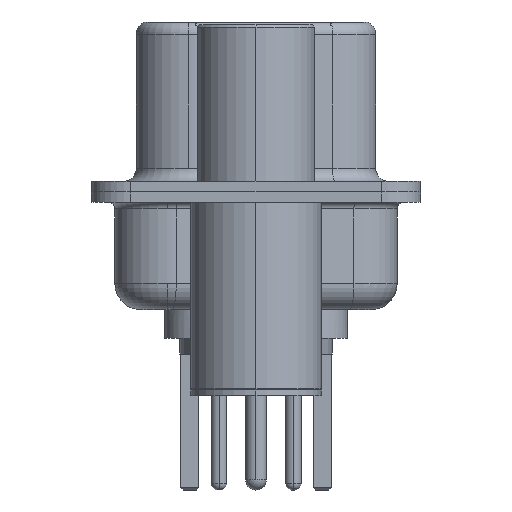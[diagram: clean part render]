
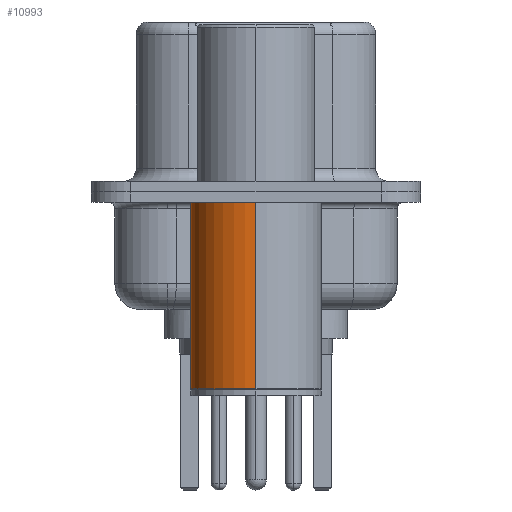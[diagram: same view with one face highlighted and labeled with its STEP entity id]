
A CAD part, left-side view. The second image highlights one B-rep face of the part: STEP entity #10993.
In plain terms, the highlighted cylindrical face has radius 2.5 mm (diameter 5 mm), a partial arc.
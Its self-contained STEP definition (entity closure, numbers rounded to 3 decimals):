
#66 = CARTESIAN_POINT ( 'NONE',  ( 0., 0., -7.525 ) ) ;
#542 = VECTOR ( 'NONE', #2726, 1000. ) ;
#605 = DIRECTION ( 'NONE',  ( 0., 0., 1. ) ) ;
#1313 = EDGE_CURVE ( 'NONE', #32355, #5717, #28626, .T. ) ;
#2302 = DIRECTION ( 'NONE',  ( 0., 0., 1. ) ) ;
#2422 = VERTEX_POINT ( 'NONE', #10895 ) ;
#2499 = ORIENTED_EDGE ( 'NONE', *, *, #11077, .F. ) ;
#2726 = DIRECTION ( 'NONE',  ( 0., 0., 1. ) ) ;
#2835 = CARTESIAN_POINT ( 'NONE',  ( 2.5, 0., -0.4 ) ) ;
#5717 = VERTEX_POINT ( 'NONE', #25246 ) ;
#5920 = LINE ( 'NONE', #27764, #12673 ) ;
#6214 = DIRECTION ( 'NONE',  ( 1., 0., 0. ) ) ;
#8095 = LINE ( 'NONE', #32632, #542 ) ;
#10231 = CYLINDRICAL_SURFACE ( 'NONE', #22922, 2.5 ) ;
#10895 = CARTESIAN_POINT ( 'NONE',  ( -2.5, 0., -0.4 ) ) ;
#10993 = ADVANCED_FACE ( 'NONE', ( #24609 ), #10231, .T. ) ;
#11077 = EDGE_CURVE ( 'NONE', #27105, #2422, #17029, .T. ) ;
#12673 = VECTOR ( 'NONE', #2302, 1000. ) ;
#12865 = EDGE_LOOP ( 'NONE', ( #32382, #17030, #2499, #18670 ) ) ;
#14269 = DIRECTION ( 'NONE',  ( 0., 0., 1. ) ) ;
#15608 = EDGE_CURVE ( 'NONE', #32355, #27105, #8095, .T. ) ;
#17029 = CIRCLE ( 'NONE', #26316, 2.5 ) ;
#17030 = ORIENTED_EDGE ( 'NONE', *, *, #19912, .T. ) ;
#18670 = ORIENTED_EDGE ( 'NONE', *, *, #15608, .F. ) ;
#19912 = EDGE_CURVE ( 'NONE', #5717, #2422, #5920, .T. ) ;
#22820 = CARTESIAN_POINT ( 'NONE',  ( 2.5, 0., -7.525 ) ) ;
#22922 = AXIS2_PLACEMENT_3D ( 'NONE', #24058, #26616, #6214 ) ;
#24058 = CARTESIAN_POINT ( 'NONE',  ( 0., 0., 0.581 ) ) ;
#24609 = FACE_OUTER_BOUND ( 'NONE', #12865, .T. ) ;
#25246 = CARTESIAN_POINT ( 'NONE',  ( -2.5, 0., -7.525 ) ) ;
#25339 = DIRECTION ( 'NONE',  ( 1., 0., 0. ) ) ;
#26316 = AXIS2_PLACEMENT_3D ( 'NONE', #29471, #14269, #32014 ) ;
#26616 = DIRECTION ( 'NONE',  ( 0., 0., 1. ) ) ;
#27105 = VERTEX_POINT ( 'NONE', #2835 ) ;
#27727 = AXIS2_PLACEMENT_3D ( 'NONE', #66, #605, #25339 ) ;
#27764 = CARTESIAN_POINT ( 'NONE',  ( -2.5, 0., 0.581 ) ) ;
#28626 = CIRCLE ( 'NONE', #27727, 2.5 ) ;
#29471 = CARTESIAN_POINT ( 'NONE',  ( 0., 0., -0.4 ) ) ;
#32014 = DIRECTION ( 'NONE',  ( 1., 0., 0. ) ) ;
#32355 = VERTEX_POINT ( 'NONE', #22820 ) ;
#32382 = ORIENTED_EDGE ( 'NONE', *, *, #1313, .T. ) ;
#32632 = CARTESIAN_POINT ( 'NONE',  ( 2.5, 0., 0.581 ) ) ;
